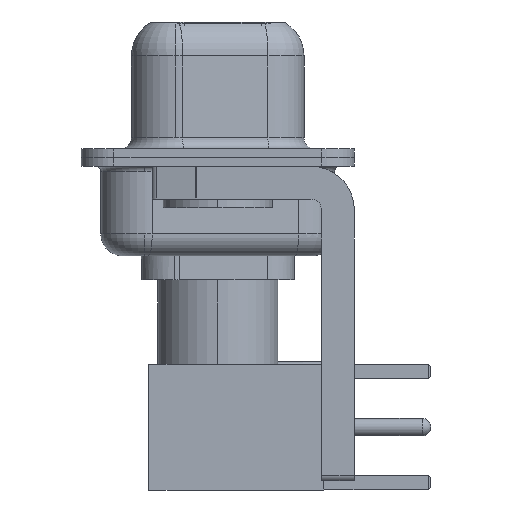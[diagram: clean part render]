
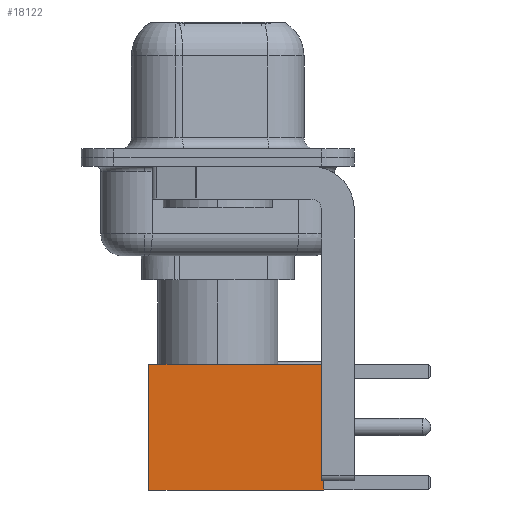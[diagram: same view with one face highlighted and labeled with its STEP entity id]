
A CAD part, left-side view. The second image highlights one B-rep face of the part: STEP entity #18122.
In plain terms, the highlighted face is planar.
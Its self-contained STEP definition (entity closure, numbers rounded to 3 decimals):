
#1158 = EDGE_CURVE ( 'NONE', #3760, #17558, #7034, .T. ) ;
#1606 = VECTOR ( 'NONE', #8314, 1000. ) ;
#2044 = VECTOR ( 'NONE', #13208, 1000. ) ;
#2110 = ORIENTED_EDGE ( 'NONE', *, *, #3030, .T. ) ;
#2627 = DIRECTION ( 'NONE',  ( 0., 0., 1. ) ) ;
#2980 = LINE ( 'NONE', #10777, #8185 ) ;
#3030 = EDGE_CURVE ( 'NONE', #17558, #6661, #14489, .T. ) ;
#3576 = CARTESIAN_POINT ( 'NONE',  ( -2.875, 2.875, 0. ) ) ;
#3760 = VERTEX_POINT ( 'NONE', #12508 ) ;
#4763 = ORIENTED_EDGE ( 'NONE', *, *, #12967, .F. ) ;
#5167 = DIRECTION ( 'NONE',  ( 0., 0., -1. ) ) ;
#5991 = VERTEX_POINT ( 'NONE', #16059 ) ;
#6606 = EDGE_CURVE ( 'NONE', #5991, #6661, #13163, .T. ) ;
#6661 = VERTEX_POINT ( 'NONE', #11457 ) ;
#7034 = LINE ( 'NONE', #16833, #1606 ) ;
#7101 = FACE_OUTER_BOUND ( 'NONE', #18648, .T. ) ;
#7425 = CARTESIAN_POINT ( 'NONE',  ( 2.875, 2.875, 0. ) ) ;
#8185 = VECTOR ( 'NONE', #17279, 1000. ) ;
#8314 = DIRECTION ( 'NONE',  ( 0., 0., -1. ) ) ;
#9597 = CARTESIAN_POINT ( 'NONE',  ( 0., 2.875, 0. ) ) ;
#10301 = PLANE ( 'NONE',  #12617 ) ;
#10777 = CARTESIAN_POINT ( 'NONE',  ( 0., 2.875, 8. ) ) ;
#11457 = CARTESIAN_POINT ( 'NONE',  ( -2.875, 2.875, 0. ) ) ;
#11990 = VECTOR ( 'NONE', #5167, 1000. ) ;
#12508 = CARTESIAN_POINT ( 'NONE',  ( 2.875, 2.875, 8. ) ) ;
#12617 = AXIS2_PLACEMENT_3D ( 'NONE', #7425, #13917, #2627 ) ;
#12967 = EDGE_CURVE ( 'NONE', #3760, #5991, #2980, .T. ) ;
#13163 = LINE ( 'NONE', #3576, #11990 ) ;
#13208 = DIRECTION ( 'NONE',  ( -1., 0., 0. ) ) ;
#13917 = DIRECTION ( 'NONE',  ( 0., 1., 0. ) ) ;
#14489 = LINE ( 'NONE', #9597, #2044 ) ;
#15696 = ORIENTED_EDGE ( 'NONE', *, *, #6606, .F. ) ;
#16042 = ORIENTED_EDGE ( 'NONE', *, *, #1158, .T. ) ;
#16059 = CARTESIAN_POINT ( 'NONE',  ( -2.875, 2.875, 8. ) ) ;
#16774 = CARTESIAN_POINT ( 'NONE',  ( 2.875, 2.875, 0. ) ) ;
#16833 = CARTESIAN_POINT ( 'NONE',  ( 2.875, 2.875, 0. ) ) ;
#17279 = DIRECTION ( 'NONE',  ( -1., 0., 0. ) ) ;
#17558 = VERTEX_POINT ( 'NONE', #16774 ) ;
#18122 = ADVANCED_FACE ( 'NONE', ( #7101 ), #10301, .T. ) ;
#18648 = EDGE_LOOP ( 'NONE', ( #16042, #2110, #15696, #4763 ) ) ;
